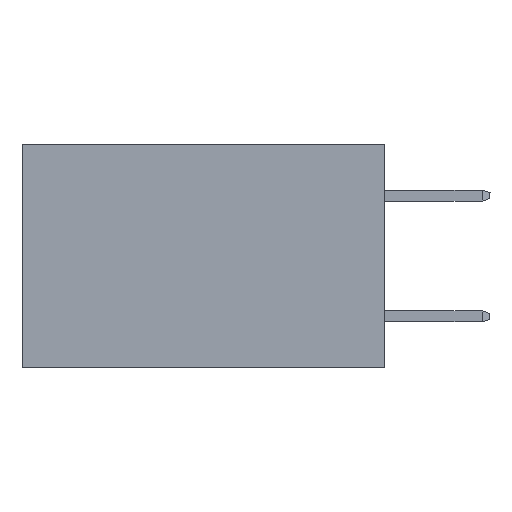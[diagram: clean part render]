
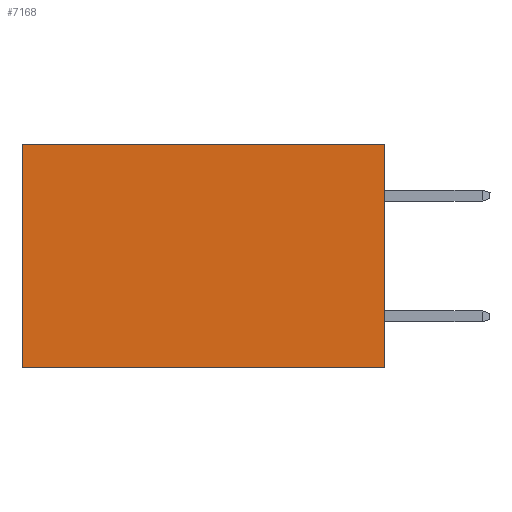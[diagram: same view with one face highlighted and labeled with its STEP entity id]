
A CAD part, left-side view. The second image highlights one B-rep face of the part: STEP entity #7168.
In plain terms, the highlighted planar face has unit normal (-1, 0, 0).
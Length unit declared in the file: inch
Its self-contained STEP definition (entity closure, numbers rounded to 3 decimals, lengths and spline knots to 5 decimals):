
#316 = EDGE_LOOP ( 'NONE', ( #9356, #8971, #30520, #3542 ) ) ;
#495 = LINE ( 'NONE', #27348, #9676 ) ;
#1847 = VERTEX_POINT ( 'NONE', #24162 ) ;
#3184 = EDGE_CURVE ( 'NONE', #7570, #1847, #495, .T. ) ;
#3542 = ORIENTED_EDGE ( 'NONE', *, *, #10338, .T. ) ;
#3816 = LINE ( 'NONE', #18612, #32915 ) ;
#6300 = LINE ( 'NONE', #16682, #18262 ) ;
#7168 = ADVANCED_FACE ( 'NONE', ( #7216 ), #18143, .F. ) ;
#7216 = FACE_OUTER_BOUND ( 'NONE', #316, .T. ) ;
#7570 = VERTEX_POINT ( 'NONE', #22561 ) ;
#8971 = ORIENTED_EDGE ( 'NONE', *, *, #19855, .F. ) ;
#9356 = ORIENTED_EDGE ( 'NONE', *, *, #13064, .T. ) ;
#9676 = VECTOR ( 'NONE', #11941, 39.37008 ) ;
#10338 = EDGE_CURVE ( 'NONE', #7570, #26904, #3816, .T. ) ;
#11941 = DIRECTION ( 'NONE',  ( 0., 0., -1. ) ) ;
#13064 = EDGE_CURVE ( 'NONE', #26904, #15612, #26340, .T. ) ;
#14815 = DIRECTION ( 'NONE',  ( 0., 0., -1. ) ) ;
#15612 = VERTEX_POINT ( 'NONE', #22517 ) ;
#16682 = CARTESIAN_POINT ( 'NONE',  ( 0.298, 0., -0.37 ) ) ;
#17252 = CARTESIAN_POINT ( 'NONE',  ( 0.298, 0., 0. ) ) ;
#18143 = PLANE ( 'NONE',  #23489 ) ;
#18262 = VECTOR ( 'NONE', #19360, 39.37008 ) ;
#18373 = CARTESIAN_POINT ( 'NONE',  ( 0.298, 0.6, 0. ) ) ;
#18390 = DIRECTION ( 'NONE',  ( 0., 1., 0. ) ) ;
#18612 = CARTESIAN_POINT ( 'NONE',  ( 0.298, 0., 0. ) ) ;
#19360 = DIRECTION ( 'NONE',  ( 0., 1., 0. ) ) ;
#19855 = EDGE_CURVE ( 'NONE', #1847, #15612, #6300, .T. ) ;
#20480 = DIRECTION ( 'NONE',  ( 0., 0., -1. ) ) ;
#22517 = CARTESIAN_POINT ( 'NONE',  ( 0.298, 0.6, -0.37 ) ) ;
#22561 = CARTESIAN_POINT ( 'NONE',  ( 0.298, 0., 0. ) ) ;
#23489 = AXIS2_PLACEMENT_3D ( 'NONE', #17252, #25602, #20480 ) ;
#24162 = CARTESIAN_POINT ( 'NONE',  ( 0.298, 0., -0.37 ) ) ;
#24291 = CARTESIAN_POINT ( 'NONE',  ( 0.298, 0.6, 0. ) ) ;
#25602 = DIRECTION ( 'NONE',  ( 1., 0., 0. ) ) ;
#25915 = VECTOR ( 'NONE', #14815, 39.37008 ) ;
#26340 = LINE ( 'NONE', #24291, #25915 ) ;
#26904 = VERTEX_POINT ( 'NONE', #18373 ) ;
#27348 = CARTESIAN_POINT ( 'NONE',  ( 0.298, 0., 0. ) ) ;
#30520 = ORIENTED_EDGE ( 'NONE', *, *, #3184, .F. ) ;
#32915 = VECTOR ( 'NONE', #18390, 39.37008 ) ;
